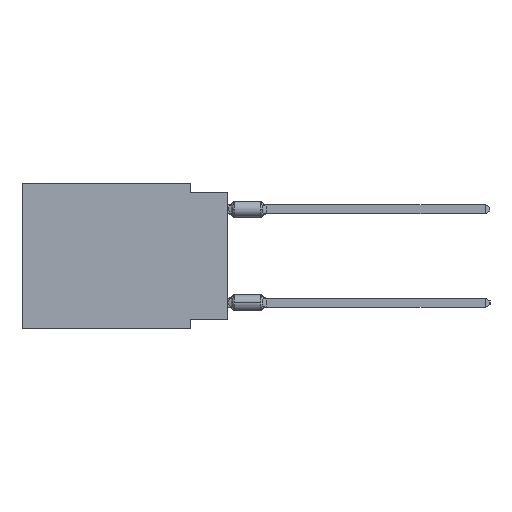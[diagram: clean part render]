
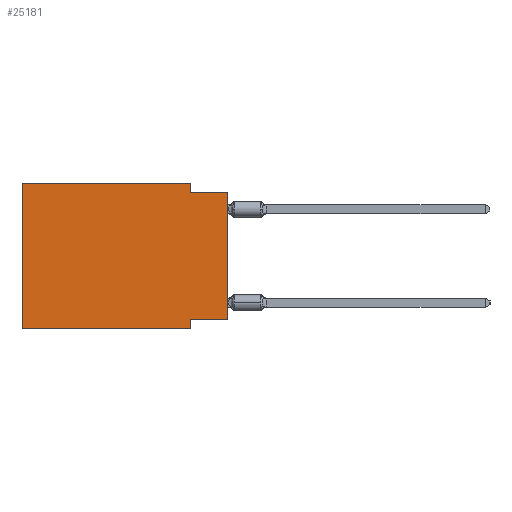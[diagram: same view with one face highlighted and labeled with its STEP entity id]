
A CAD part, left-side view. The second image highlights one B-rep face of the part: STEP entity #25181.
In plain terms, the highlighted planar face has unit normal (-1, 0, 0).
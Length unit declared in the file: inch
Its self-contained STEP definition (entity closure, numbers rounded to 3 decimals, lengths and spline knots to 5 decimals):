
#324 = DIRECTION ( 'NONE',  ( 0., 0., 1. ) ) ;
#1117 = EDGE_CURVE ( 'NONE', #8442, #3526, #22164, .T. ) ;
#1870 = VECTOR ( 'NONE', #6386, 39.37008 ) ;
#2991 = VERTEX_POINT ( 'NONE', #11559 ) ;
#3423 = AXIS2_PLACEMENT_3D ( 'NONE', #46378, #46658, #10663 ) ;
#3526 = VERTEX_POINT ( 'NONE', #13821 ) ;
#4709 = CARTESIAN_POINT ( 'NONE',  ( 0., 0., -0.025 ) ) ;
#4955 = VECTOR ( 'NONE', #324, 39.37008 ) ;
#5253 = EDGE_CURVE ( 'NONE', #3526, #6642, #17447, .T. ) ;
#5400 = CARTESIAN_POINT ( 'NONE',  ( 0., 0., 0. ) ) ;
#5468 = ORIENTED_EDGE ( 'NONE', *, *, #31554, .F. ) ;
#6386 = DIRECTION ( 'NONE',  ( 0., 1., 0. ) ) ;
#6642 = VERTEX_POINT ( 'NONE', #25197 ) ;
#8442 = VERTEX_POINT ( 'NONE', #51679 ) ;
#10023 = LINE ( 'NONE', #33683, #1870 ) ;
#10663 = DIRECTION ( 'NONE',  ( 0., 0., -1. ) ) ;
#11115 = LINE ( 'NONE', #29988, #52448 ) ;
#11559 = CARTESIAN_POINT ( 'NONE',  ( 0., 0., -0.365 ) ) ;
#13821 = CARTESIAN_POINT ( 'NONE',  ( 0., 0.1, 0. ) ) ;
#14985 = CARTESIAN_POINT ( 'NONE',  ( 0., 0.1, -0.39 ) ) ;
#17213 = DIRECTION ( 'NONE',  ( 0., -1., 0. ) ) ;
#17267 = DIRECTION ( 'NONE',  ( 0., -1., 0. ) ) ;
#17447 = LINE ( 'NONE', #22245, #47288 ) ;
#18106 = EDGE_CURVE ( 'NONE', #2991, #25080, #41998, .T. ) ;
#18277 = CARTESIAN_POINT ( 'NONE',  ( 0., 0.55, 0. ) ) ;
#19080 = FACE_OUTER_BOUND ( 'NONE', #27428, .T. ) ;
#20612 = CARTESIAN_POINT ( 'NONE',  ( 0., 0.1, -0.365 ) ) ;
#20862 = ORIENTED_EDGE ( 'NONE', *, *, #41536, .T. ) ;
#22164 = LINE ( 'NONE', #18277, #29149 ) ;
#22245 = CARTESIAN_POINT ( 'NONE',  ( 0., 0.1, 0. ) ) ;
#22271 = EDGE_CURVE ( 'NONE', #6642, #25080, #45735, .T. ) ;
#25080 = VERTEX_POINT ( 'NONE', #4709 ) ;
#25181 = ADVANCED_FACE ( 'NONE', ( #19080 ), #51724, .F. ) ;
#25197 = CARTESIAN_POINT ( 'NONE',  ( 0., 0.1, -0.025 ) ) ;
#26451 = DIRECTION ( 'NONE',  ( 0., 0., -1. ) ) ;
#26993 = ORIENTED_EDGE ( 'NONE', *, *, #32015, .F. ) ;
#27428 = EDGE_LOOP ( 'NONE', ( #35783, #40986, #47411, #37139, #47304, #20862, #5468, #26993 ) ) ;
#28511 = VERTEX_POINT ( 'NONE', #20612 ) ;
#29149 = VECTOR ( 'NONE', #54523, 39.37008 ) ;
#29815 = EDGE_CURVE ( 'NONE', #52225, #8442, #11115, .T. ) ;
#29988 = CARTESIAN_POINT ( 'NONE',  ( 0., 0.55, 0. ) ) ;
#31554 = EDGE_CURVE ( 'NONE', #28511, #47508, #56033, .T. ) ;
#32015 = EDGE_CURVE ( 'NONE', #2991, #28511, #10023, .T. ) ;
#33683 = CARTESIAN_POINT ( 'NONE',  ( 0., 0., -0.365 ) ) ;
#34281 = CARTESIAN_POINT ( 'NONE',  ( 0., 0.1, -0.39 ) ) ;
#35783 = ORIENTED_EDGE ( 'NONE', *, *, #18106, .T. ) ;
#36130 = CARTESIAN_POINT ( 'NONE',  ( 0., 0., -0.025 ) ) ;
#37139 = ORIENTED_EDGE ( 'NONE', *, *, #1117, .F. ) ;
#37827 = DIRECTION ( 'NONE',  ( 0., 0., 1. ) ) ;
#39198 = VECTOR ( 'NONE', #43726, 39.37008 ) ;
#40079 = LINE ( 'NONE', #58313, #42025 ) ;
#40986 = ORIENTED_EDGE ( 'NONE', *, *, #22271, .F. ) ;
#41536 = EDGE_CURVE ( 'NONE', #52225, #47508, #40079, .T. ) ;
#41998 = LINE ( 'NONE', #5400, #4955 ) ;
#42025 = VECTOR ( 'NONE', #17267, 39.37008 ) ;
#43726 = DIRECTION ( 'NONE',  ( 0., 0., -1. ) ) ;
#44369 = CARTESIAN_POINT ( 'NONE',  ( 0., 0.55, -0.39 ) ) ;
#45735 = LINE ( 'NONE', #36130, #57736 ) ;
#46378 = CARTESIAN_POINT ( 'NONE',  ( 0., 0.55, 0. ) ) ;
#46658 = DIRECTION ( 'NONE',  ( 1., 0., 0. ) ) ;
#47288 = VECTOR ( 'NONE', #26451, 39.37008 ) ;
#47304 = ORIENTED_EDGE ( 'NONE', *, *, #29815, .F. ) ;
#47411 = ORIENTED_EDGE ( 'NONE', *, *, #5253, .F. ) ;
#47508 = VERTEX_POINT ( 'NONE', #34281 ) ;
#51679 = CARTESIAN_POINT ( 'NONE',  ( 0., 0.55, 0. ) ) ;
#51724 = PLANE ( 'NONE',  #3423 ) ;
#52225 = VERTEX_POINT ( 'NONE', #44369 ) ;
#52448 = VECTOR ( 'NONE', #37827, 39.37008 ) ;
#54523 = DIRECTION ( 'NONE',  ( 0., -1., 0. ) ) ;
#56033 = LINE ( 'NONE', #14985, #39198 ) ;
#57736 = VECTOR ( 'NONE', #17213, 39.37008 ) ;
#58313 = CARTESIAN_POINT ( 'NONE',  ( 0., 0.55, -0.39 ) ) ;
